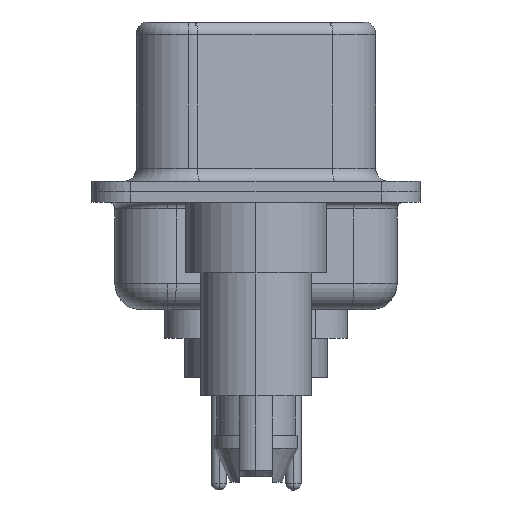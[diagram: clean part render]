
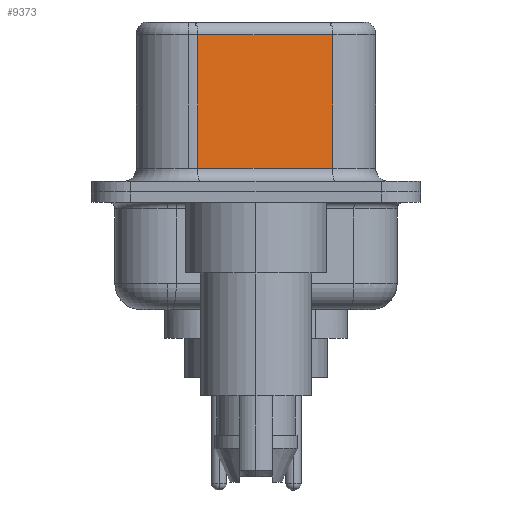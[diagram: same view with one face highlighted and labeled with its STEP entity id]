
A CAD part, left-side view. The second image highlights one B-rep face of the part: STEP entity #9373.
In plain terms, the highlighted planar face has unit normal (-0.985, -0.174, 0).
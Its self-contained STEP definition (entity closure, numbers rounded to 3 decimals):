
#328 = ORIENTED_EDGE ( 'NONE', *, *, #12835, .F. ) ;
#409 = DIRECTION ( 'NONE',  ( -0.174, 0.985, 0. ) ) ;
#568 = DIRECTION ( 'NONE',  ( 0., 0., -1. ) ) ;
#586 = EDGE_CURVE ( 'NONE', #13850, #20000, #21392, .T. ) ;
#769 = LINE ( 'NONE', #21305, #13960 ) ;
#3193 = VECTOR ( 'NONE', #20023, 1000. ) ;
#4313 = ORIENTED_EDGE ( 'NONE', *, *, #18112, .T. ) ;
#6068 = CARTESIAN_POINT ( 'NONE',  ( 4.58, -2.927, 6.52 ) ) ;
#6127 = CARTESIAN_POINT ( 'NONE',  ( 3.67, 2.233, 6.02 ) ) ;
#7692 = CARTESIAN_POINT ( 'NONE',  ( 4.58, -2.927, 6.02 ) ) ;
#8147 = CARTESIAN_POINT ( 'NONE',  ( 4.58, -2.927, 0.9 ) ) ;
#8476 = VERTEX_POINT ( 'NONE', #11431 ) ;
#8995 = PLANE ( 'NONE',  #16710 ) ;
#9373 = ADVANCED_FACE ( 'NONE', ( #16308 ), #8995, .F. ) ;
#10143 = ORIENTED_EDGE ( 'NONE', *, *, #586, .T. ) ;
#10434 = CARTESIAN_POINT ( 'NONE',  ( 4.58, -2.927, 6.02 ) ) ;
#10734 = DIRECTION ( 'NONE',  ( 0.985, 0.174, 0. ) ) ;
#11360 = CARTESIAN_POINT ( 'NONE',  ( 4.58, -2.927, 0.9 ) ) ;
#11431 = CARTESIAN_POINT ( 'NONE',  ( 3.67, 2.233, 0.9 ) ) ;
#12112 = VECTOR ( 'NONE', #15257, 1000. ) ;
#12379 = LINE ( 'NONE', #11360, #3193 ) ;
#12448 = VERTEX_POINT ( 'NONE', #8147 ) ;
#12835 = EDGE_CURVE ( 'NONE', #13850, #12448, #20298, .T. ) ;
#13732 = EDGE_LOOP ( 'NONE', ( #328, #10143, #21692, #4313 ) ) ;
#13850 = VERTEX_POINT ( 'NONE', #10434 ) ;
#13960 = VECTOR ( 'NONE', #568, 1000. ) ;
#15257 = DIRECTION ( 'NONE',  ( -0.174, 0.985, 0. ) ) ;
#16308 = FACE_OUTER_BOUND ( 'NONE', #13732, .T. ) ;
#16432 = DIRECTION ( 'NONE',  ( 0., 0., -1. ) ) ;
#16710 = AXIS2_PLACEMENT_3D ( 'NONE', #17628, #10734, #409 ) ;
#17628 = CARTESIAN_POINT ( 'NONE',  ( 4.58, -2.927, 6.52 ) ) ;
#18112 = EDGE_CURVE ( 'NONE', #8476, #12448, #12379, .T. ) ;
#19745 = VECTOR ( 'NONE', #16432, 1000. ) ;
#19831 = EDGE_CURVE ( 'NONE', #20000, #8476, #769, .T. ) ;
#20000 = VERTEX_POINT ( 'NONE', #6127 ) ;
#20023 = DIRECTION ( 'NONE',  ( 0.174, -0.985, 0. ) ) ;
#20298 = LINE ( 'NONE', #6068, #19745 ) ;
#21305 = CARTESIAN_POINT ( 'NONE',  ( 3.67, 2.233, 6.52 ) ) ;
#21392 = LINE ( 'NONE', #7692, #12112 ) ;
#21692 = ORIENTED_EDGE ( 'NONE', *, *, #19831, .T. ) ;
